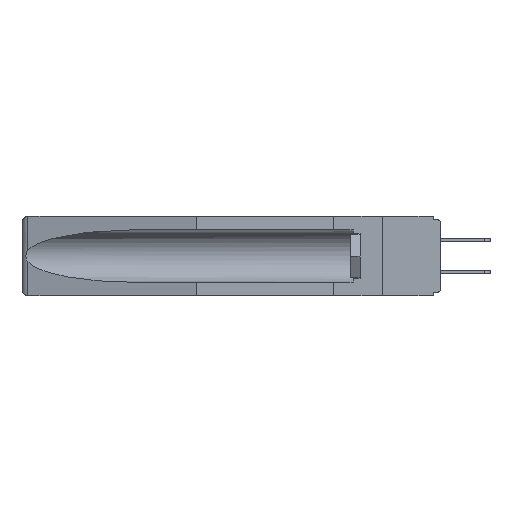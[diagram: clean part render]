
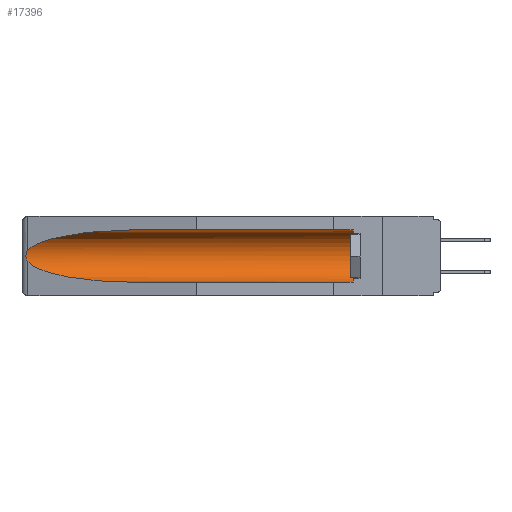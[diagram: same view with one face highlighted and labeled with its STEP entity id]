
A CAD part, left-side view. The second image highlights one B-rep face of the part: STEP entity #17396.
In plain terms, the highlighted cylindrical face has radius 2.857 mm (diameter 5.715 mm), a partial arc.
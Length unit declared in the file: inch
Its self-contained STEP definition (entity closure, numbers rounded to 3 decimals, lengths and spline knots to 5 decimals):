
#231 = EDGE_CURVE ( 'NONE', #254, #8230, #7679, .T. ) ;
#254 = VERTEX_POINT ( 'NONE', #1183 ) ;
#491 = VERTEX_POINT ( 'NONE', #1314 ) ;
#677 = FACE_OUTER_BOUND ( 'NONE', #10585, .T. ) ;
#696 = DIRECTION ( 'NONE',  ( 0., 0., 1. ) ) ;
#914 = AXIS2_PLACEMENT_3D ( 'NONE', #9759, #1670, #19483 ) ;
#1032 = CARTESIAN_POINT ( 'NONE',  ( 0.26655, 1.53094, -0.18657 ) ) ;
#1183 = CARTESIAN_POINT ( 'NONE',  ( 0.26537, 1.52718, -0.14972 ) ) ;
#1314 = CARTESIAN_POINT ( 'NONE',  ( 0.155, 1.07973, -0.059 ) ) ;
#1368 = EDGE_CURVE ( 'NONE', #8230, #7743, #11065, .T. ) ;
#1670 = DIRECTION ( 'NONE',  ( 0., 1., 0. ) ) ;
#2659 = CARTESIAN_POINT ( 'NONE',  ( 0.2673, 1.53269, -0.17917 ) ) ;
#2856 = LINE ( 'NONE', #9799, #11730 ) ;
#3275 =( BOUNDED_CURVE ( )  B_SPLINE_CURVE ( 3, ( #6139, #20814, #20743, #17430 ),
 .UNSPECIFIED., .F., .F. ) 
 B_SPLINE_CURVE_WITH_KNOTS ( ( 4, 4 ),
 ( 4.71239, 6.08839 ),
 .UNSPECIFIED. ) 
 CURVE ( )  GEOMETRIC_REPRESENTATION_ITEM ( )  RATIONAL_B_SPLINE_CURVE ( ( 1., 0.848, 0.848, 1. ) ) 
 REPRESENTATION_ITEM ( '' )  );
#3933 = VERTEX_POINT ( 'NONE', #4295 ) ;
#4269 = CARTESIAN_POINT ( 'NONE',  ( 0.26537, 1.52718, -0.19328 ) ) ;
#4295 = CARTESIAN_POINT ( 'NONE',  ( 0.155, 0.126, -0.059 ) ) ;
#5666 = EDGE_CURVE ( 'NONE', #7127, #3933, #13523, .T. ) ;
#5798 = CARTESIAN_POINT ( 'NONE',  ( 0.2675, 1.53308, -0.17534 ) ) ;
#5866 = CARTESIAN_POINT ( 'NONE',  ( 0.2673, 1.5327, -0.16383 ) ) ;
#6006 = CARTESIAN_POINT ( 'NONE',  ( 0.26597, 1.5296, -0.19026 ) ) ;
#6139 = CARTESIAN_POINT ( 'NONE',  ( 0.155, 1.07973, -0.059 ) ) ;
#6174 = EDGE_CURVE ( 'NONE', #3933, #491, #7675, .T. ) ;
#6538 = ORIENTED_EDGE ( 'NONE', *, *, #231, .T. ) ;
#6556 = ORIENTED_EDGE ( 'NONE', *, *, #5666, .T. ) ;
#7127 = VERTEX_POINT ( 'NONE', #12656 ) ;
#7146 = DIRECTION ( 'NONE',  ( 0., -1., 0. ) ) ;
#7639 = CARTESIAN_POINT ( 'NONE',  ( 0.155, 1.07973, -0.284 ) ) ;
#7675 = LINE ( 'NONE', #17393, #17511 ) ;
#7679 = B_SPLINE_CURVE_WITH_KNOTS ( 'NONE', 3,
 ( #12233, #12386, #20538, #5866, #15485, #5798, #2659, #1032, #6006, #4269 ),
 .UNSPECIFIED., .F., .F.,
 ( 4, 2, 2, 2, 4 ),
 ( 0., 0.00029, 0.00058, 0.00087, 0.00117 ),
 .UNSPECIFIED. ) ;
#7743 = VERTEX_POINT ( 'NONE', #7639 ) ;
#8230 = VERTEX_POINT ( 'NONE', #17283 ) ;
#9212 = CARTESIAN_POINT ( 'NONE',  ( 0.21114, 1.30732, -0.284 ) ) ;
#9759 = CARTESIAN_POINT ( 'NONE',  ( 0.155, -0.30754, -0.1715 ) ) ;
#9799 = CARTESIAN_POINT ( 'NONE',  ( 0.155, -0.30754, -0.284 ) ) ;
#10192 = ORIENTED_EDGE ( 'NONE', *, *, #12831, .F. ) ;
#10240 = CARTESIAN_POINT ( 'NONE',  ( 0.155, 0.126, -0.1715 ) ) ;
#10585 = EDGE_LOOP ( 'NONE', ( #12002, #6538, #15121, #10192, #6556, #11052 ) ) ;
#11052 = ORIENTED_EDGE ( 'NONE', *, *, #6174, .T. ) ;
#11065 =( BOUNDED_CURVE ( )  B_SPLINE_CURVE ( 3, ( #14191, #20625, #9212, #12617 ),
 .UNSPECIFIED., .F., .F. ) 
 B_SPLINE_CURVE_WITH_KNOTS ( ( 4, 4 ),
 ( 0.1948, 1.5708 ),
 .UNSPECIFIED. ) 
 CURVE ( )  GEOMETRIC_REPRESENTATION_ITEM ( )  RATIONAL_B_SPLINE_CURVE ( ( 1., 0.848, 0.848, 1. ) ) 
 REPRESENTATION_ITEM ( '' )  );
#11539 = EDGE_CURVE ( 'NONE', #491, #254, #3275, .T. ) ;
#11730 = VECTOR ( 'NONE', #16089, 39.37008 ) ;
#12002 = ORIENTED_EDGE ( 'NONE', *, *, #11539, .T. ) ;
#12233 = CARTESIAN_POINT ( 'NONE',  ( 0.26537, 1.52718, -0.14972 ) ) ;
#12386 = CARTESIAN_POINT ( 'NONE',  ( 0.26597, 1.52961, -0.15275 ) ) ;
#12617 = CARTESIAN_POINT ( 'NONE',  ( 0.155, 1.07973, -0.284 ) ) ;
#12656 = CARTESIAN_POINT ( 'NONE',  ( 0.155, 0.126, -0.284 ) ) ;
#12831 = EDGE_CURVE ( 'NONE', #7127, #7743, #2856, .T. ) ;
#13523 = CIRCLE ( 'NONE', #15604, 0.1125 ) ;
#14191 = CARTESIAN_POINT ( 'NONE',  ( 0.26537, 1.52718, -0.19328 ) ) ;
#14665 = CYLINDRICAL_SURFACE ( 'NONE', #914, 0.1125 ) ;
#15121 = ORIENTED_EDGE ( 'NONE', *, *, #1368, .T. ) ;
#15485 = CARTESIAN_POINT ( 'NONE',  ( 0.2675, 1.53308, -0.16763 ) ) ;
#15604 = AXIS2_PLACEMENT_3D ( 'NONE', #10240, #7146, #696 ) ;
#16089 = DIRECTION ( 'NONE',  ( 0., 1., 0. ) ) ;
#17283 = CARTESIAN_POINT ( 'NONE',  ( 0.26537, 1.52718, -0.19328 ) ) ;
#17393 = CARTESIAN_POINT ( 'NONE',  ( 0.155, -0.30754, -0.059 ) ) ;
#17396 = ADVANCED_FACE ( 'NONE', ( #677 ), #14665, .F. ) ;
#17430 = CARTESIAN_POINT ( 'NONE',  ( 0.26537, 1.52718, -0.14972 ) ) ;
#17511 = VECTOR ( 'NONE', #19007, 39.37008 ) ;
#19007 = DIRECTION ( 'NONE',  ( 0., 1., 0. ) ) ;
#19483 = DIRECTION ( 'NONE',  ( 0., 0., 1. ) ) ;
#20538 = CARTESIAN_POINT ( 'NONE',  ( 0.26654, 1.53092, -0.15636 ) ) ;
#20625 = CARTESIAN_POINT ( 'NONE',  ( 0.25451, 1.48313, -0.24835 ) ) ;
#20743 = CARTESIAN_POINT ( 'NONE',  ( 0.25451, 1.48313, -0.09465 ) ) ;
#20814 = CARTESIAN_POINT ( 'NONE',  ( 0.21114, 1.30732, -0.059 ) ) ;
